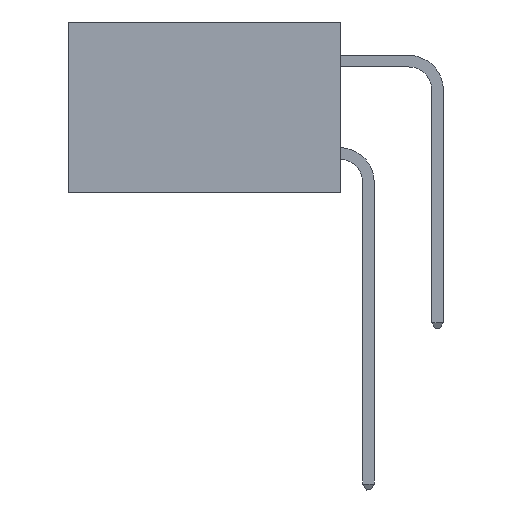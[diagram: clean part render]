
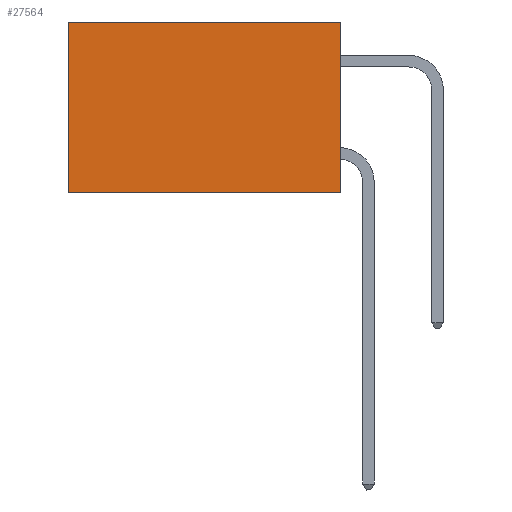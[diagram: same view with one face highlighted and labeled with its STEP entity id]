
A CAD part, left-side view. The second image highlights one B-rep face of the part: STEP entity #27564.
In plain terms, the highlighted planar face has unit normal (-1, 0, 0).
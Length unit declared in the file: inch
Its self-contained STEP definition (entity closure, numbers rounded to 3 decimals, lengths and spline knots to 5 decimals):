
#548 = CARTESIAN_POINT ( 'NONE',  ( 0.277, 0., 0. ) ) ;
#1376 = CARTESIAN_POINT ( 'NONE',  ( 0.277, 0.59, -0.37 ) ) ;
#1885 = VERTEX_POINT ( 'NONE', #548 ) ;
#3571 = FACE_OUTER_BOUND ( 'NONE', #8563, .T. ) ;
#3701 = VERTEX_POINT ( 'NONE', #20359 ) ;
#4220 = CARTESIAN_POINT ( 'NONE',  ( 0.277, 0., -0.37 ) ) ;
#5231 = VERTEX_POINT ( 'NONE', #24929 ) ;
#6035 = AXIS2_PLACEMENT_3D ( 'NONE', #11929, #26781, #14054 ) ;
#6460 = DIRECTION ( 'NONE',  ( 0., 1., 0. ) ) ;
#6903 = VERTEX_POINT ( 'NONE', #1376 ) ;
#6911 = CARTESIAN_POINT ( 'NONE',  ( 0.277, 0., -0.37 ) ) ;
#7941 = ORIENTED_EDGE ( 'NONE', *, *, #20827, .T. ) ;
#8405 = VECTOR ( 'NONE', #21966, 39.37008 ) ;
#8563 = EDGE_LOOP ( 'NONE', ( #7941, #20724, #9106, #19806 ) ) ;
#9106 = ORIENTED_EDGE ( 'NONE', *, *, #27401, .F. ) ;
#11929 = CARTESIAN_POINT ( 'NONE',  ( 0.277, 0., -0.37 ) ) ;
#14054 = DIRECTION ( 'NONE',  ( 0., 0., -1. ) ) ;
#14553 = EDGE_CURVE ( 'NONE', #1885, #3701, #26719, .T. ) ;
#16091 = VECTOR ( 'NONE', #19789, 39.37008 ) ;
#16188 = LINE ( 'NONE', #20758, #26815 ) ;
#18183 = VECTOR ( 'NONE', #6460, 39.37008 ) ;
#19766 = EDGE_CURVE ( 'NONE', #5231, #6903, #23847, .T. ) ;
#19789 = DIRECTION ( 'NONE',  ( 0., 1., 0. ) ) ;
#19791 = LINE ( 'NONE', #6911, #8405 ) ;
#19806 = ORIENTED_EDGE ( 'NONE', *, *, #14553, .T. ) ;
#20359 = CARTESIAN_POINT ( 'NONE',  ( 0.277, 0.59, 0. ) ) ;
#20366 = PLANE ( 'NONE',  #6035 ) ;
#20724 = ORIENTED_EDGE ( 'NONE', *, *, #19766, .F. ) ;
#20758 = CARTESIAN_POINT ( 'NONE',  ( 0.277, 0.59, -0.37 ) ) ;
#20827 = EDGE_CURVE ( 'NONE', #3701, #6903, #16188, .T. ) ;
#21966 = DIRECTION ( 'NONE',  ( 0., 0., -1. ) ) ;
#22917 = DIRECTION ( 'NONE',  ( 0., 0., -1. ) ) ;
#23847 = LINE ( 'NONE', #4220, #18183 ) ;
#24929 = CARTESIAN_POINT ( 'NONE',  ( 0.277, 0., -0.37 ) ) ;
#26128 = CARTESIAN_POINT ( 'NONE',  ( 0.277, 0., 0. ) ) ;
#26719 = LINE ( 'NONE', #26128, #16091 ) ;
#26781 = DIRECTION ( 'NONE',  ( 1., 0., 0. ) ) ;
#26815 = VECTOR ( 'NONE', #22917, 39.37008 ) ;
#27401 = EDGE_CURVE ( 'NONE', #1885, #5231, #19791, .T. ) ;
#27564 = ADVANCED_FACE ( 'NONE', ( #3571 ), #20366, .F. ) ;
